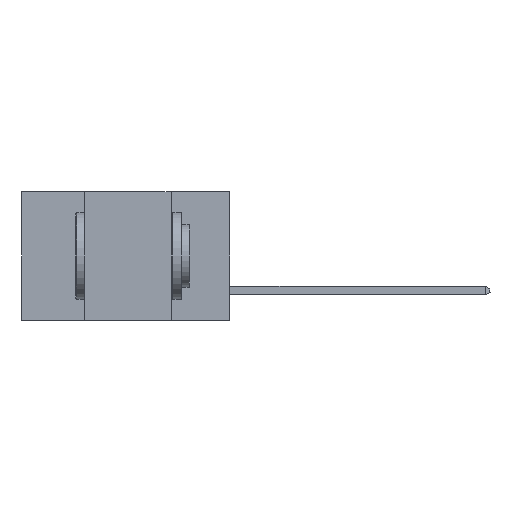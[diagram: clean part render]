
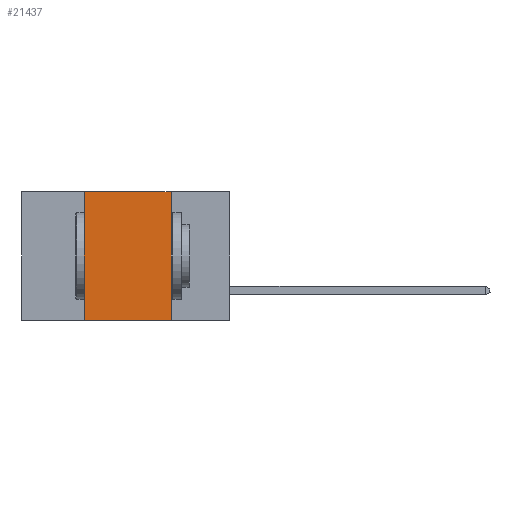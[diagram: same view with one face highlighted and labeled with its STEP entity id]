
A CAD part, left-side view. The second image highlights one B-rep face of the part: STEP entity #21437.
In plain terms, the highlighted planar face has unit normal (-1, 0, 0).
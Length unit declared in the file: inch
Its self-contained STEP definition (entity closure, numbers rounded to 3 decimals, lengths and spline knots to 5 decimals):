
#53 = VECTOR ( 'NONE', #17715, 39.37008 ) ;
#259 = EDGE_CURVE ( 'NONE', #9890, #16077, #10006, .T. ) ;
#696 = ORIENTED_EDGE ( 'NONE', *, *, #259, .T. ) ;
#994 = EDGE_LOOP ( 'NONE', ( #1456, #20346, #19696, #696 ) ) ;
#1456 = ORIENTED_EDGE ( 'NONE', *, *, #19370, .F. ) ;
#1460 = LINE ( 'NONE', #11653, #2002 ) ;
#1541 = DIRECTION ( 'NONE',  ( 0., 0., 1. ) ) ;
#2002 = VECTOR ( 'NONE', #1541, 39.37008 ) ;
#2065 = VECTOR ( 'NONE', #9821, 39.37008 ) ;
#2177 = LINE ( 'NONE', #5910, #53 ) ;
#5311 = FACE_OUTER_BOUND ( 'NONE', #994, .T. ) ;
#5910 = CARTESIAN_POINT ( 'NONE',  ( 0., 0.17, 0. ) ) ;
#7072 = PLANE ( 'NONE',  #19416 ) ;
#7145 = CARTESIAN_POINT ( 'NONE',  ( 0., 0.17, -0.37 ) ) ;
#7372 = LINE ( 'NONE', #16649, #2065 ) ;
#7780 = VERTEX_POINT ( 'NONE', #11514 ) ;
#8054 = VERTEX_POINT ( 'NONE', #17136 ) ;
#8559 = DIRECTION ( 'NONE',  ( 1., 0., 0. ) ) ;
#8829 = EDGE_CURVE ( 'NONE', #8054, #7780, #7372, .T. ) ;
#8994 = CARTESIAN_POINT ( 'NONE',  ( 0., 0.42, -0.37 ) ) ;
#9821 = DIRECTION ( 'NONE',  ( 0., -1., 0. ) ) ;
#9890 = VERTEX_POINT ( 'NONE', #8994 ) ;
#10006 = LINE ( 'NONE', #13887, #10262 ) ;
#10262 = VECTOR ( 'NONE', #15661, 39.37008 ) ;
#11514 = CARTESIAN_POINT ( 'NONE',  ( 0., 0.17, 0. ) ) ;
#11653 = CARTESIAN_POINT ( 'NONE',  ( 0., 0.42, 0. ) ) ;
#13887 = CARTESIAN_POINT ( 'NONE',  ( 0., 0.6, -0.37 ) ) ;
#15661 = DIRECTION ( 'NONE',  ( 0., -1., 0. ) ) ;
#16077 = VERTEX_POINT ( 'NONE', #7145 ) ;
#16649 = CARTESIAN_POINT ( 'NONE',  ( 0., 0.6, 0. ) ) ;
#17136 = CARTESIAN_POINT ( 'NONE',  ( 0., 0.42, 0. ) ) ;
#17715 = DIRECTION ( 'NONE',  ( 0., 0., -1. ) ) ;
#17903 = EDGE_CURVE ( 'NONE', #9890, #8054, #1460, .T. ) ;
#19370 = EDGE_CURVE ( 'NONE', #7780, #16077, #2177, .T. ) ;
#19416 = AXIS2_PLACEMENT_3D ( 'NONE', #20631, #8559, #20408 ) ;
#19696 = ORIENTED_EDGE ( 'NONE', *, *, #17903, .F. ) ;
#20346 = ORIENTED_EDGE ( 'NONE', *, *, #8829, .F. ) ;
#20408 = DIRECTION ( 'NONE',  ( 0., 0., -1. ) ) ;
#20631 = CARTESIAN_POINT ( 'NONE',  ( 0., 0.6, 0. ) ) ;
#21437 = ADVANCED_FACE ( 'NONE', ( #5311 ), #7072, .F. ) ;
